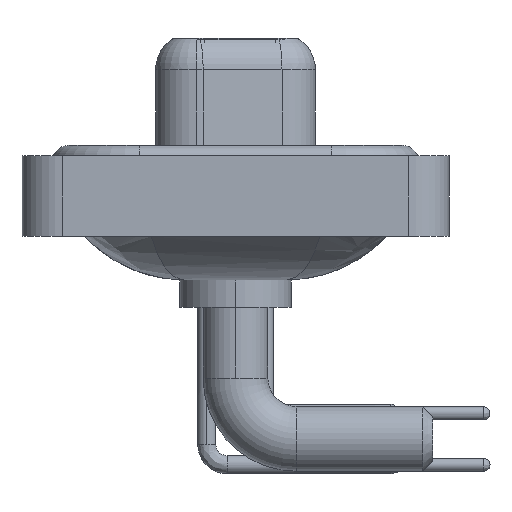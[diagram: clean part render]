
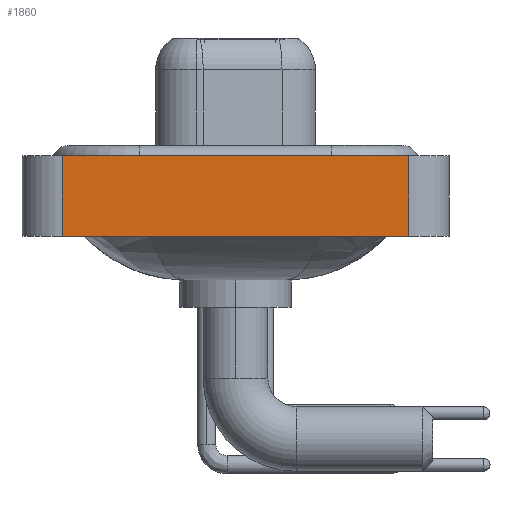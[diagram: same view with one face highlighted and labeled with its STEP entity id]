
A CAD part, left-side view. The second image highlights one B-rep face of the part: STEP entity #1860.
In plain terms, the highlighted planar face has unit normal (-1, 0, 0).
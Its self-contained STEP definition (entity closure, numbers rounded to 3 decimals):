
#603 = DIRECTION ( 'NONE',  ( 0., 0., 1. ) ) ;
#942 = DIRECTION ( 'NONE',  ( 0., 0., 1. ) ) ;
#1584 = DIRECTION ( 'NONE',  ( 0., -1., 0. ) ) ;
#1860 = ADVANCED_FACE ( 'NONE', ( #5411 ), #12227, .T. ) ;
#2160 = ORIENTED_EDGE ( 'NONE', *, *, #7347, .F. ) ;
#2269 = CARTESIAN_POINT ( 'NONE',  ( -7.35, -8.55, -3.6 ) ) ;
#3826 = VECTOR ( 'NONE', #942, 1000. ) ;
#4334 = AXIS2_PLACEMENT_3D ( 'NONE', #13479, #9035, #603 ) ;
#5411 = FACE_OUTER_BOUND ( 'NONE', #12354, .T. ) ;
#5566 = CARTESIAN_POINT ( 'NONE',  ( -7.35, 8.55, -3.6 ) ) ;
#5668 = EDGE_CURVE ( 'NONE', #19318, #17944, #18803, .T. ) ;
#6282 = ORIENTED_EDGE ( 'NONE', *, *, #5668, .F. ) ;
#7017 = DIRECTION ( 'NONE',  ( 0., -1., 0. ) ) ;
#7347 = EDGE_CURVE ( 'NONE', #17944, #13834, #14550, .T. ) ;
#9035 = DIRECTION ( 'NONE',  ( -1., 0., 0. ) ) ;
#9547 = VECTOR ( 'NONE', #1584, 1000. ) ;
#10797 = ORIENTED_EDGE ( 'NONE', *, *, #19175, .T. ) ;
#12227 = PLANE ( 'NONE',  #4334 ) ;
#12354 = EDGE_LOOP ( 'NONE', ( #10797, #2160, #6282, #20446 ) ) ;
#12400 = CARTESIAN_POINT ( 'NONE',  ( -7.35, -8.55, 0.4 ) ) ;
#12921 = LINE ( 'NONE', #19375, #19834 ) ;
#13403 = LINE ( 'NONE', #16904, #13977 ) ;
#13479 = CARTESIAN_POINT ( 'NONE',  ( -7.35, -8.55, -3.6 ) ) ;
#13834 = VERTEX_POINT ( 'NONE', #12400 ) ;
#13977 = VECTOR ( 'NONE', #7017, 1000. ) ;
#14550 = LINE ( 'NONE', #16256, #9547 ) ;
#15605 = EDGE_CURVE ( 'NONE', #19318, #19311, #13403, .T. ) ;
#16256 = CARTESIAN_POINT ( 'NONE',  ( -7.35, -8.55, 0.4 ) ) ;
#16902 = CARTESIAN_POINT ( 'NONE',  ( -7.35, 8.55, 0.4 ) ) ;
#16904 = CARTESIAN_POINT ( 'NONE',  ( -7.35, -8.55, -3.6 ) ) ;
#17112 = CARTESIAN_POINT ( 'NONE',  ( -7.35, 8.55, -3.6 ) ) ;
#17778 = DIRECTION ( 'NONE',  ( 0., 0., 1. ) ) ;
#17944 = VERTEX_POINT ( 'NONE', #16902 ) ;
#18803 = LINE ( 'NONE', #17112, #3826 ) ;
#19175 = EDGE_CURVE ( 'NONE', #19311, #13834, #12921, .T. ) ;
#19311 = VERTEX_POINT ( 'NONE', #2269 ) ;
#19318 = VERTEX_POINT ( 'NONE', #5566 ) ;
#19375 = CARTESIAN_POINT ( 'NONE',  ( -7.35, -8.55, -3.6 ) ) ;
#19834 = VECTOR ( 'NONE', #17778, 1000. ) ;
#20446 = ORIENTED_EDGE ( 'NONE', *, *, #15605, .T. ) ;
